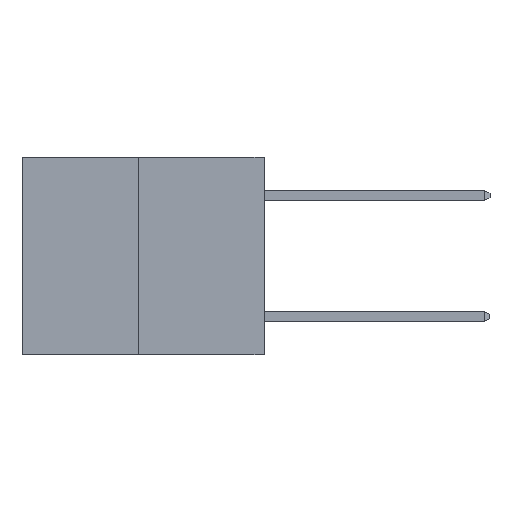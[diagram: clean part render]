
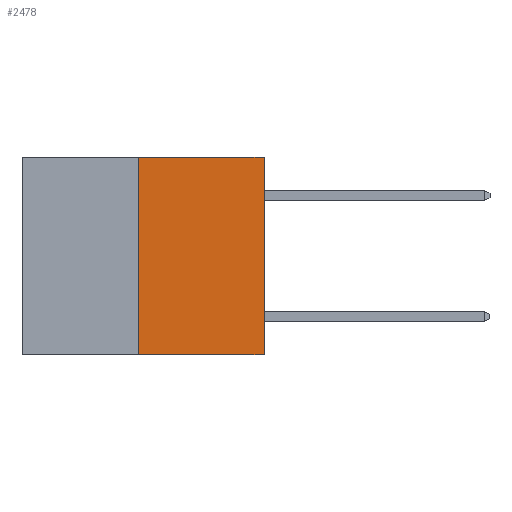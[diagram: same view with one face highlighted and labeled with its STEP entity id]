
A CAD part, left-side view. The second image highlights one B-rep face of the part: STEP entity #2478.
In plain terms, the highlighted planar face has unit normal (-1, 0, 0).
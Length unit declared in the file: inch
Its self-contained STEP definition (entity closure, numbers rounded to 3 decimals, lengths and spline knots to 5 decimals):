
#4 = LINE ( 'NONE', #5758, #9963 ) ;
#203 = CARTESIAN_POINT ( 'NONE',  ( 0., 0.312, -0.49 ) ) ;
#352 = EDGE_CURVE ( 'NONE', #8373, #8755, #5526, .T. ) ;
#1144 = CARTESIAN_POINT ( 'NONE',  ( 0., 0., 0. ) ) ;
#1479 = CARTESIAN_POINT ( 'NONE',  ( 0., 0.312, 0. ) ) ;
#1559 = EDGE_CURVE ( 'NONE', #11734, #7724, #3718, .T. ) ;
#1670 = CARTESIAN_POINT ( 'NONE',  ( 0., 0.312, -0.49 ) ) ;
#2048 = CARTESIAN_POINT ( 'NONE',  ( 0., 0.6, 0. ) ) ;
#2112 = EDGE_CURVE ( 'NONE', #7724, #8755, #6092, .T. ) ;
#2183 = DIRECTION ( 'NONE',  ( 0., 0., 1. ) ) ;
#2478 = ADVANCED_FACE ( 'NONE', ( #10232 ), #10607, .F. ) ;
#3718 = LINE ( 'NONE', #203, #9797 ) ;
#4113 = AXIS2_PLACEMENT_3D ( 'NONE', #4493, #11661, #5530 ) ;
#4493 = CARTESIAN_POINT ( 'NONE',  ( 0., 0.6, 0. ) ) ;
#4692 = ORIENTED_EDGE ( 'NONE', *, *, #2112, .F. ) ;
#4943 = CARTESIAN_POINT ( 'NONE',  ( 0., 0., 0. ) ) ;
#5526 = LINE ( 'NONE', #1144, #10163 ) ;
#5530 = DIRECTION ( 'NONE',  ( 0., 0., -1. ) ) ;
#5758 = CARTESIAN_POINT ( 'NONE',  ( 0., 0.6, -0.49 ) ) ;
#6092 = LINE ( 'NONE', #2048, #6411 ) ;
#6411 = VECTOR ( 'NONE', #11317, 39.37008 ) ;
#7144 = ORIENTED_EDGE ( 'NONE', *, *, #7899, .T. ) ;
#7724 = VERTEX_POINT ( 'NONE', #1479 ) ;
#7899 = EDGE_CURVE ( 'NONE', #11734, #8373, #4, .T. ) ;
#8253 = DIRECTION ( 'NONE',  ( 0., 0., 1. ) ) ;
#8373 = VERTEX_POINT ( 'NONE', #11183 ) ;
#8755 = VERTEX_POINT ( 'NONE', #4943 ) ;
#9441 = ORIENTED_EDGE ( 'NONE', *, *, #352, .T. ) ;
#9797 = VECTOR ( 'NONE', #8253, 39.37008 ) ;
#9963 = VECTOR ( 'NONE', #10930, 39.37008 ) ;
#10163 = VECTOR ( 'NONE', #2183, 39.37008 ) ;
#10232 = FACE_OUTER_BOUND ( 'NONE', #13048, .T. ) ;
#10514 = ORIENTED_EDGE ( 'NONE', *, *, #1559, .F. ) ;
#10607 = PLANE ( 'NONE',  #4113 ) ;
#10930 = DIRECTION ( 'NONE',  ( 0., -1., 0. ) ) ;
#11183 = CARTESIAN_POINT ( 'NONE',  ( 0., 0., -0.49 ) ) ;
#11317 = DIRECTION ( 'NONE',  ( 0., -1., 0. ) ) ;
#11661 = DIRECTION ( 'NONE',  ( 1., 0., 0. ) ) ;
#11734 = VERTEX_POINT ( 'NONE', #1670 ) ;
#13048 = EDGE_LOOP ( 'NONE', ( #10514, #7144, #9441, #4692 ) ) ;
